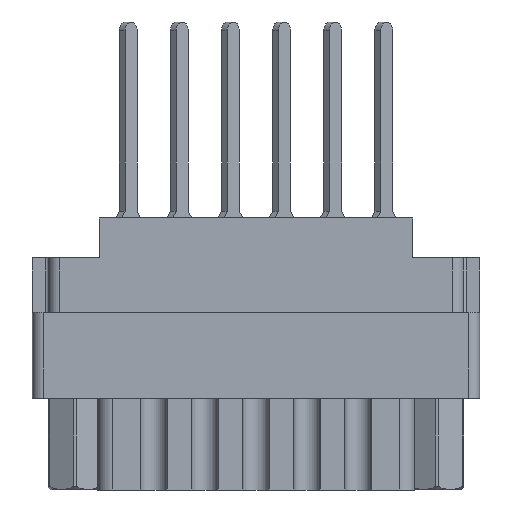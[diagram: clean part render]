
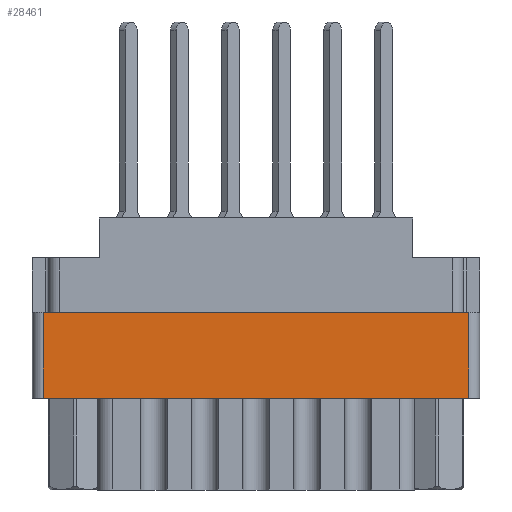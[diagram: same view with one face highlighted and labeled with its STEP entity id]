
A CAD part, front view. The second image highlights one B-rep face of the part: STEP entity #28461.
In plain terms, the highlighted planar face has unit normal (0, -1, 0).
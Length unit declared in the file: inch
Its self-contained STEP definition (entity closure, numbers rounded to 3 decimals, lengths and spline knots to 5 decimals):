
#754 = CARTESIAN_POINT ( 'NONE',  ( -0.624, -0.343, -0.798 ) ) ;
#3180 = CARTESIAN_POINT ( 'NONE',  ( 0.624, -0.343, -0.798 ) ) ;
#3546 = DIRECTION ( 'NONE',  ( 0., -1., 0. ) ) ;
#3722 = FACE_OUTER_BOUND ( 'NONE', #12490, .T. ) ;
#4793 = VECTOR ( 'NONE', #13716, 39.37008 ) ;
#5477 = LINE ( 'NONE', #17488, #16033 ) ;
#7658 = VERTEX_POINT ( 'NONE', #16770 ) ;
#7899 = VECTOR ( 'NONE', #16662, 39.37008 ) ;
#7908 = EDGE_CURVE ( 'NONE', #15471, #25806, #5477, .T. ) ;
#8957 = CARTESIAN_POINT ( 'NONE',  ( -0.624, -0.343, -0.277 ) ) ;
#11100 = LINE ( 'NONE', #23874, #7899 ) ;
#12490 = EDGE_LOOP ( 'NONE', ( #13494, #24683, #29130, #27055 ) ) ;
#12887 = DIRECTION ( 'NONE',  ( 1., 0., 0. ) ) ;
#13279 = PLANE ( 'NONE',  #31092 ) ;
#13494 = ORIENTED_EDGE ( 'NONE', *, *, #27364, .F. ) ;
#13604 = DIRECTION ( 'NONE',  ( 0., 0., -1. ) ) ;
#13716 = DIRECTION ( 'NONE',  ( 0., 0., 1. ) ) ;
#15411 = CARTESIAN_POINT ( 'NONE',  ( 0.624, -0.343, -0.529 ) ) ;
#15471 = VERTEX_POINT ( 'NONE', #8957 ) ;
#16033 = VECTOR ( 'NONE', #12887, 39.37008 ) ;
#16662 = DIRECTION ( 'NONE',  ( -1., 0., 0. ) ) ;
#16770 = CARTESIAN_POINT ( 'NONE',  ( -0.624, -0.343, -0.529 ) ) ;
#16923 = VECTOR ( 'NONE', #17470, 39.37008 ) ;
#17109 = CARTESIAN_POINT ( 'NONE',  ( 0.624, -0.343, -0.277 ) ) ;
#17306 = CARTESIAN_POINT ( 'NONE',  ( -0.624, -0.343, -0.798 ) ) ;
#17470 = DIRECTION ( 'NONE',  ( 0., 0., 1. ) ) ;
#17488 = CARTESIAN_POINT ( 'NONE',  ( -0.656, -0.343, -0.277 ) ) ;
#17934 = LINE ( 'NONE', #17306, #16923 ) ;
#22184 = EDGE_CURVE ( 'NONE', #28331, #7658, #11100, .T. ) ;
#23874 = CARTESIAN_POINT ( 'NONE',  ( 0.624, -0.343, -0.529 ) ) ;
#24683 = ORIENTED_EDGE ( 'NONE', *, *, #22184, .F. ) ;
#25806 = VERTEX_POINT ( 'NONE', #17109 ) ;
#26560 = EDGE_CURVE ( 'NONE', #28331, #25806, #28615, .T. ) ;
#27055 = ORIENTED_EDGE ( 'NONE', *, *, #7908, .F. ) ;
#27364 = EDGE_CURVE ( 'NONE', #7658, #15471, #17934, .T. ) ;
#28331 = VERTEX_POINT ( 'NONE', #15411 ) ;
#28461 = ADVANCED_FACE ( 'NONE', ( #3722 ), #13279, .T. ) ;
#28615 = LINE ( 'NONE', #3180, #4793 ) ;
#29130 = ORIENTED_EDGE ( 'NONE', *, *, #26560, .T. ) ;
#31092 = AXIS2_PLACEMENT_3D ( 'NONE', #754, #3546, #13604 ) ;
